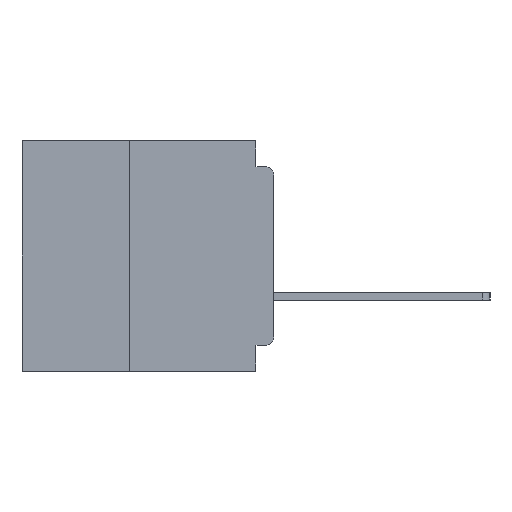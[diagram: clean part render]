
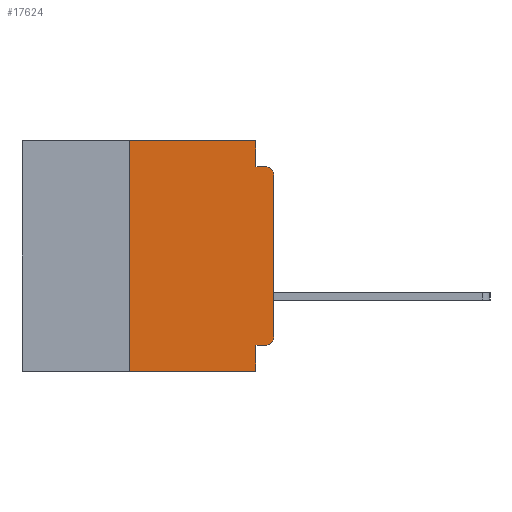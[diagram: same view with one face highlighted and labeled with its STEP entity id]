
A CAD part, left-side view. The second image highlights one B-rep face of the part: STEP entity #17624.
In plain terms, the highlighted planar face has unit normal (-1, 0, 0).
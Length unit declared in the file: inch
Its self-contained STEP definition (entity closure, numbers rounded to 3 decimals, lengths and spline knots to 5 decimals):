
#156 = LINE ( 'NONE', #29715, #30397 ) ;
#246 = DIRECTION ( 'NONE',  ( 0., 1., 0. ) ) ;
#2057 = CARTESIAN_POINT ( 'NONE',  ( 0., 0.015, -0.355 ) ) ;
#2153 = ORIENTED_EDGE ( 'NONE', *, *, #8479, .T. ) ;
#2398 = VECTOR ( 'NONE', #26172, 39.37008 ) ;
#2695 = EDGE_CURVE ( 'NONE', #21385, #34140, #14449, .T. ) ;
#2977 = ORIENTED_EDGE ( 'NONE', *, *, #2695, .F. ) ;
#3606 = CARTESIAN_POINT ( 'NONE',  ( 0., 0.437, 0. ) ) ;
#3977 = DIRECTION ( 'NONE',  ( 0., 0., 1. ) ) ;
#4860 = VECTOR ( 'NONE', #246, 39.37008 ) ;
#5362 = LINE ( 'NONE', #6892, #27846 ) ;
#5787 = DIRECTION ( 'NONE',  ( -1., 0., 0. ) ) ;
#5811 = LINE ( 'NONE', #24458, #29198 ) ;
#6156 = AXIS2_PLACEMENT_3D ( 'NONE', #14859, #35411, #17809 ) ;
#6892 = CARTESIAN_POINT ( 'NONE',  ( 0., 0., 0. ) ) ;
#7121 = VERTEX_POINT ( 'NONE', #31526 ) ;
#7184 = CARTESIAN_POINT ( 'NONE',  ( 0., 0., -0.06 ) ) ;
#8137 = ORIENTED_EDGE ( 'NONE', *, *, #30180, .F. ) ;
#8479 = EDGE_CURVE ( 'NONE', #10851, #10096, #26129, .T. ) ;
#9859 = CARTESIAN_POINT ( 'NONE',  ( 0., 0.25, 0. ) ) ;
#10096 = VERTEX_POINT ( 'NONE', #10241 ) ;
#10241 = CARTESIAN_POINT ( 'NONE',  ( 0., 0., -0.34 ) ) ;
#10851 = VERTEX_POINT ( 'NONE', #2057 ) ;
#11263 = ORIENTED_EDGE ( 'NONE', *, *, #22535, .T. ) ;
#12396 = PLANE ( 'NONE',  #13779 ) ;
#12768 = DIRECTION ( 'NONE',  ( 0., 0., -1. ) ) ;
#13779 = AXIS2_PLACEMENT_3D ( 'NONE', #3606, #15341, #35898 ) ;
#13832 = DIRECTION ( 'NONE',  ( 0., 0., 1. ) ) ;
#14317 = CARTESIAN_POINT ( 'NONE',  ( 0., 0., -0.045 ) ) ;
#14427 = EDGE_CURVE ( 'NONE', #37970, #34140, #156, .T. ) ;
#14449 = LINE ( 'NONE', #22476, #20437 ) ;
#14730 = ORIENTED_EDGE ( 'NONE', *, *, #20358, .F. ) ;
#14859 = CARTESIAN_POINT ( 'NONE',  ( 0., 0.015, -0.06 ) ) ;
#15288 = FACE_OUTER_BOUND ( 'NONE', #26758, .T. ) ;
#15341 = DIRECTION ( 'NONE',  ( 1., 0., 0. ) ) ;
#16039 = VECTOR ( 'NONE', #13832, 39.37008 ) ;
#17624 = ADVANCED_FACE ( 'NONE', ( #15288 ), #12396, .F. ) ;
#17809 = DIRECTION ( 'NONE',  ( 0., 0., -1. ) ) ;
#17950 = LINE ( 'NONE', #14317, #2398 ) ;
#18008 = DIRECTION ( 'NONE',  ( 0., -1., 0. ) ) ;
#18497 = CARTESIAN_POINT ( 'NONE',  ( 0., 0.25, -0.4 ) ) ;
#19719 = ORIENTED_EDGE ( 'NONE', *, *, #25460, .F. ) ;
#19750 = CARTESIAN_POINT ( 'NONE',  ( 0., 0.25, -0.4 ) ) ;
#20346 = ORIENTED_EDGE ( 'NONE', *, *, #14427, .T. ) ;
#20358 = EDGE_CURVE ( 'NONE', #37970, #33462, #23861, .T. ) ;
#20437 = VECTOR ( 'NONE', #26048, 39.37008 ) ;
#21385 = VERTEX_POINT ( 'NONE', #36346 ) ;
#21409 = VECTOR ( 'NONE', #31245, 39.37008 ) ;
#22209 = VERTEX_POINT ( 'NONE', #28872 ) ;
#22476 = CARTESIAN_POINT ( 'NONE',  ( 0., 0.031, -0.4 ) ) ;
#22535 = EDGE_CURVE ( 'NONE', #10096, #29595, #5362, .T. ) ;
#23324 = CARTESIAN_POINT ( 'NONE',  ( 0., 0.015, -0.34 ) ) ;
#23861 = LINE ( 'NONE', #19750, #16039 ) ;
#24458 = CARTESIAN_POINT ( 'NONE',  ( 0., 0.031, 0. ) ) ;
#25460 = EDGE_CURVE ( 'NONE', #33462, #7121, #29246, .T. ) ;
#26048 = DIRECTION ( 'NONE',  ( 0., 0., -1. ) ) ;
#26129 = CIRCLE ( 'NONE', #34928, 0.015 ) ;
#26172 = DIRECTION ( 'NONE',  ( 0., -1., 0. ) ) ;
#26231 = EDGE_CURVE ( 'NONE', #29595, #22209, #27835, .T. ) ;
#26314 = DIRECTION ( 'NONE',  ( 0., 0., -1. ) ) ;
#26758 = EDGE_LOOP ( 'NONE', ( #11263, #33790, #29265, #8137, #19719, #14730, #20346, #2977, #30097, #2153 ) ) ;
#27449 = VERTEX_POINT ( 'NONE', #37994 ) ;
#27835 = CIRCLE ( 'NONE', #6156, 0.015 ) ;
#27846 = VECTOR ( 'NONE', #3977, 39.37008 ) ;
#28872 = CARTESIAN_POINT ( 'NONE',  ( 0., 0.015, -0.045 ) ) ;
#29160 = LINE ( 'NONE', #29584, #4860 ) ;
#29198 = VECTOR ( 'NONE', #12768, 39.37008 ) ;
#29246 = LINE ( 'NONE', #37021, #21409 ) ;
#29265 = ORIENTED_EDGE ( 'NONE', *, *, #32602, .F. ) ;
#29584 = CARTESIAN_POINT ( 'NONE',  ( 0., 0., -0.355 ) ) ;
#29595 = VERTEX_POINT ( 'NONE', #7184 ) ;
#29715 = CARTESIAN_POINT ( 'NONE',  ( 0., 0.437, -0.4 ) ) ;
#30097 = ORIENTED_EDGE ( 'NONE', *, *, #30634, .F. ) ;
#30180 = EDGE_CURVE ( 'NONE', #7121, #27449, #5811, .T. ) ;
#30397 = VECTOR ( 'NONE', #18008, 39.37008 ) ;
#30634 = EDGE_CURVE ( 'NONE', #10851, #21385, #29160, .T. ) ;
#31245 = DIRECTION ( 'NONE',  ( 0., -1., 0. ) ) ;
#31526 = CARTESIAN_POINT ( 'NONE',  ( 0., 0.031, 0. ) ) ;
#32602 = EDGE_CURVE ( 'NONE', #27449, #22209, #17950, .T. ) ;
#33462 = VERTEX_POINT ( 'NONE', #9859 ) ;
#33790 = ORIENTED_EDGE ( 'NONE', *, *, #26231, .T. ) ;
#34140 = VERTEX_POINT ( 'NONE', #36290 ) ;
#34928 = AXIS2_PLACEMENT_3D ( 'NONE', #23324, #5787, #26314 ) ;
#35411 = DIRECTION ( 'NONE',  ( -1., 0., 0. ) ) ;
#35898 = DIRECTION ( 'NONE',  ( 0., 0., -1. ) ) ;
#36290 = CARTESIAN_POINT ( 'NONE',  ( 0., 0.031, -0.4 ) ) ;
#36346 = CARTESIAN_POINT ( 'NONE',  ( 0., 0.031, -0.355 ) ) ;
#37021 = CARTESIAN_POINT ( 'NONE',  ( 0., 0.437, 0. ) ) ;
#37970 = VERTEX_POINT ( 'NONE', #18497 ) ;
#37994 = CARTESIAN_POINT ( 'NONE',  ( 0., 0.031, -0.045 ) ) ;
